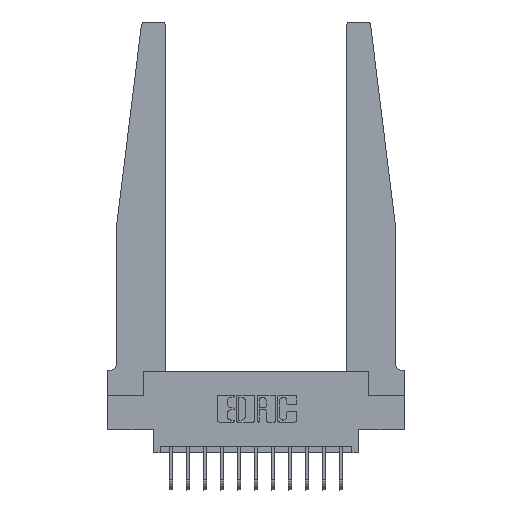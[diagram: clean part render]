
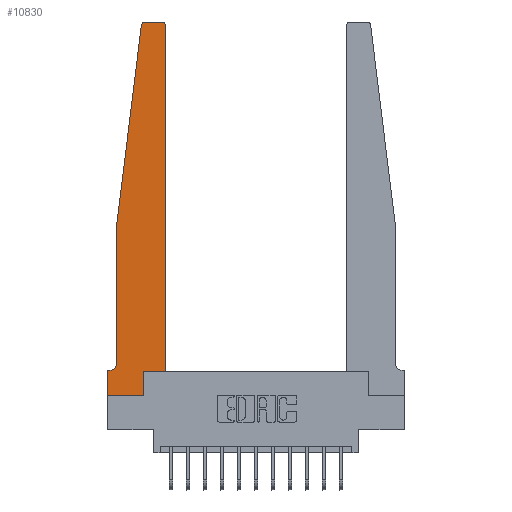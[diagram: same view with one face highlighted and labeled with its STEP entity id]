
A CAD part, top view. The second image highlights one B-rep face of the part: STEP entity #10830.
In plain terms, the highlighted planar face has unit normal (0, 0, 1).
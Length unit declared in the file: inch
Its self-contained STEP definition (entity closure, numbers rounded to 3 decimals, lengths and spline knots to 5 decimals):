
#116 = ORIENTED_EDGE ( 'NONE', *, *, #6315, .T. ) ;
#223 = EDGE_CURVE ( 'NONE', #5155, #6280, #10210, .T. ) ;
#361 = AXIS2_PLACEMENT_3D ( 'NONE', #9776, #11028, #3672 ) ;
#482 = ORIENTED_EDGE ( 'NONE', *, *, #3084, .T. ) ;
#535 = VERTEX_POINT ( 'NONE', #7776 ) ;
#606 = CARTESIAN_POINT ( 'NONE',  ( 0.395, 2.75, 0.37 ) ) ;
#818 = VECTOR ( 'NONE', #10014, 39.37008 ) ;
#1107 = PLANE ( 'NONE',  #361 ) ;
#1334 = CARTESIAN_POINT ( 'NONE',  ( 0., 0., 0.37 ) ) ;
#1417 = EDGE_CURVE ( 'NONE', #2126, #9722, #3248, .T. ) ;
#1606 = VECTOR ( 'NONE', #13996, 39.37008 ) ;
#1800 = EDGE_CURVE ( 'NONE', #8484, #535, #9396, .T. ) ;
#1886 = CARTESIAN_POINT ( 'NONE',  ( 0., 0.1875, 0.37 ) ) ;
#2126 = VERTEX_POINT ( 'NONE', #1886 ) ;
#2200 = ORIENTED_EDGE ( 'NONE', *, *, #5519, .T. ) ;
#2440 = EDGE_LOOP ( 'NONE', ( #116, #14006, #482, #8449, #13731, #2200, #14453, #2810, #8343, #15510, #6123, #3665 ) ) ;
#2810 = ORIENTED_EDGE ( 'NONE', *, *, #6102, .T. ) ;
#3084 = EDGE_CURVE ( 'NONE', #5366, #14981, #10704, .T. ) ;
#3248 = LINE ( 'NONE', #5738, #9411 ) ;
#3665 = ORIENTED_EDGE ( 'NONE', *, *, #5190, .T. ) ;
#3672 = DIRECTION ( 'NONE',  ( 1., 0., 0. ) ) ;
#3702 = CARTESIAN_POINT ( 'NONE',  ( 0.065, 1.25, 0.37 ) ) ;
#3898 = VECTOR ( 'NONE', #12754, 39.37008 ) ;
#4389 = VECTOR ( 'NONE', #6929, 39.37008 ) ;
#4601 = DIRECTION ( 'NONE',  ( -1., 0., 0. ) ) ;
#4683 = CIRCLE ( 'NONE', #9890, 0.03 ) ;
#4763 = DIRECTION ( 'NONE',  ( 0., 0., -1. ) ) ;
#4906 = VECTOR ( 'NONE', #14692, 39.37008 ) ;
#5155 = VERTEX_POINT ( 'NONE', #10044 ) ;
#5190 = EDGE_CURVE ( 'NONE', #15928, #10523, #4683, .T. ) ;
#5207 = CARTESIAN_POINT ( 'NONE',  ( 0.395, 2.72, 0.37 ) ) ;
#5292 = EDGE_CURVE ( 'NONE', #535, #15928, #12149, .T. ) ;
#5366 = VERTEX_POINT ( 'NONE', #5513 ) ;
#5452 = CARTESIAN_POINT ( 'NONE',  ( 0.065, 1.25, 0.37 ) ) ;
#5463 = CARTESIAN_POINT ( 'NONE',  ( 0.425, 0.18, 0.37 ) ) ;
#5513 = CARTESIAN_POINT ( 'NONE',  ( 0.24675, 2.72367, 0.37 ) ) ;
#5519 = EDGE_CURVE ( 'NONE', #6280, #2126, #12344, .T. ) ;
#5584 = CARTESIAN_POINT ( 'NONE',  ( 0.015, 0.1875, 0.37 ) ) ;
#5738 = CARTESIAN_POINT ( 'NONE',  ( 0., 0., 0.37 ) ) ;
#6102 = EDGE_CURVE ( 'NONE', #9722, #12919, #13575, .T. ) ;
#6123 = ORIENTED_EDGE ( 'NONE', *, *, #5292, .T. ) ;
#6149 = VECTOR ( 'NONE', #7888, 39.37008 ) ;
#6222 = VECTOR ( 'NONE', #4601, 39.37008 ) ;
#6280 = VERTEX_POINT ( 'NONE', #5584 ) ;
#6315 = EDGE_CURVE ( 'NONE', #10523, #12380, #7665, .T. ) ;
#6446 = DIRECTION ( 'NONE',  ( 1., 0., 0. ) ) ;
#6883 = CARTESIAN_POINT ( 'NONE',  ( 0.25, 2.75, 0.37 ) ) ;
#6929 = DIRECTION ( 'NONE',  ( -1., 0., 0. ) ) ;
#6986 = DIRECTION ( 'NONE',  ( 0., -1., 0. ) ) ;
#7421 = DIRECTION ( 'NONE',  ( 0., 0., 1. ) ) ;
#7665 = LINE ( 'NONE', #6883, #4389 ) ;
#7776 = CARTESIAN_POINT ( 'NONE',  ( 0.425, 0.18, 0.37 ) ) ;
#7880 = CARTESIAN_POINT ( 'NONE',  ( 0.065, 1.25, 0.37 ) ) ;
#7888 = DIRECTION ( 'NONE',  ( 1., 0., 0. ) ) ;
#8061 = EDGE_CURVE ( 'NONE', #14981, #5155, #11446, .T. ) ;
#8090 = CIRCLE ( 'NONE', #13293, 0.03 ) ;
#8343 = ORIENTED_EDGE ( 'NONE', *, *, #14344, .T. ) ;
#8449 = ORIENTED_EDGE ( 'NONE', *, *, #8061, .T. ) ;
#8484 = VERTEX_POINT ( 'NONE', #11820 ) ;
#9396 = LINE ( 'NONE', #12937, #6149 ) ;
#9411 = VECTOR ( 'NONE', #6986, 39.37008 ) ;
#9722 = VERTEX_POINT ( 'NONE', #14360 ) ;
#9776 = CARTESIAN_POINT ( 'NONE',  ( 0., 0.1875, 0.37 ) ) ;
#9890 = AXIS2_PLACEMENT_3D ( 'NONE', #5207, #13749, #6446 ) ;
#10014 = DIRECTION ( 'NONE',  ( 1., 0., 0. ) ) ;
#10044 = CARTESIAN_POINT ( 'NONE',  ( 0.065, 0.2375, 0.37 ) ) ;
#10210 = CIRCLE ( 'NONE', #14398, 0.05 ) ;
#10523 = VERTEX_POINT ( 'NONE', #606 ) ;
#10704 = LINE ( 'NONE', #5452, #1606 ) ;
#10830 = ADVANCED_FACE ( 'NONE', ( #15139 ), #1107, .T. ) ;
#11028 = DIRECTION ( 'NONE',  ( 0., 0., 1. ) ) ;
#11217 = CARTESIAN_POINT ( 'NONE',  ( 0.425, 2.72, 0.37 ) ) ;
#11446 = LINE ( 'NONE', #3702, #4906 ) ;
#11450 = EDGE_CURVE ( 'NONE', #12380, #5366, #8090, .T. ) ;
#11540 = CARTESIAN_POINT ( 'NONE',  ( 0.2605, 0.18, 0.37 ) ) ;
#11820 = CARTESIAN_POINT ( 'NONE',  ( 0.2605, 0.18, 0.37 ) ) ;
#11931 = CARTESIAN_POINT ( 'NONE',  ( 0.065, 0.1875, 0.37 ) ) ;
#12089 = CARTESIAN_POINT ( 'NONE',  ( 0.015, 0.2375, 0.37 ) ) ;
#12149 = LINE ( 'NONE', #5463, #15765 ) ;
#12344 = LINE ( 'NONE', #11931, #6222 ) ;
#12380 = VERTEX_POINT ( 'NONE', #15109 ) ;
#12754 = DIRECTION ( 'NONE',  ( 0., 1., 0. ) ) ;
#12919 = VERTEX_POINT ( 'NONE', #15099 ) ;
#12937 = CARTESIAN_POINT ( 'NONE',  ( 0.425, 0.18, 0.37 ) ) ;
#13293 = AXIS2_PLACEMENT_3D ( 'NONE', #14710, #7421, #15955 ) ;
#13300 = DIRECTION ( 'NONE',  ( -1., 0., 0. ) ) ;
#13575 = LINE ( 'NONE', #1334, #818 ) ;
#13645 = LINE ( 'NONE', #11540, #3898 ) ;
#13731 = ORIENTED_EDGE ( 'NONE', *, *, #223, .T. ) ;
#13749 = DIRECTION ( 'NONE',  ( 0., 0., 1. ) ) ;
#13996 = DIRECTION ( 'NONE',  ( -0.122, -0.992, 0. ) ) ;
#14006 = ORIENTED_EDGE ( 'NONE', *, *, #11450, .T. ) ;
#14009 = DIRECTION ( 'NONE',  ( 0., 1., 0. ) ) ;
#14344 = EDGE_CURVE ( 'NONE', #12919, #8484, #13645, .T. ) ;
#14360 = CARTESIAN_POINT ( 'NONE',  ( 0., 0., 0.37 ) ) ;
#14398 = AXIS2_PLACEMENT_3D ( 'NONE', #12089, #4763, #13300 ) ;
#14453 = ORIENTED_EDGE ( 'NONE', *, *, #1417, .T. ) ;
#14692 = DIRECTION ( 'NONE',  ( 0., -1., 0. ) ) ;
#14710 = CARTESIAN_POINT ( 'NONE',  ( 0.27653, 2.72, 0.37 ) ) ;
#14981 = VERTEX_POINT ( 'NONE', #7880 ) ;
#15099 = CARTESIAN_POINT ( 'NONE',  ( 0.2605, 0., 0.37 ) ) ;
#15109 = CARTESIAN_POINT ( 'NONE',  ( 0.27653, 2.75, 0.37 ) ) ;
#15139 = FACE_OUTER_BOUND ( 'NONE', #2440, .T. ) ;
#15510 = ORIENTED_EDGE ( 'NONE', *, *, #1800, .T. ) ;
#15765 = VECTOR ( 'NONE', #14009, 39.37008 ) ;
#15928 = VERTEX_POINT ( 'NONE', #11217 ) ;
#15955 = DIRECTION ( 'NONE',  ( 1., 0., 0. ) ) ;
